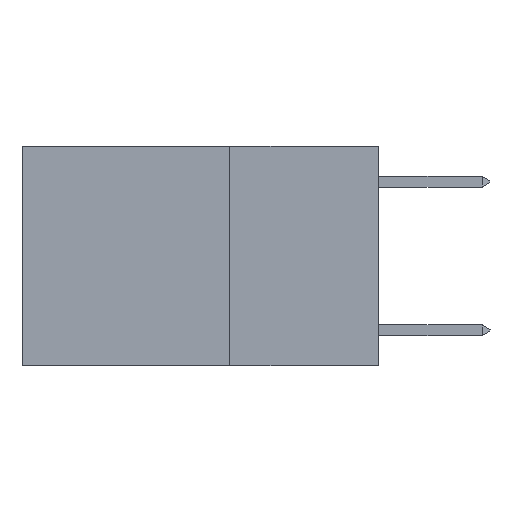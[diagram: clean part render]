
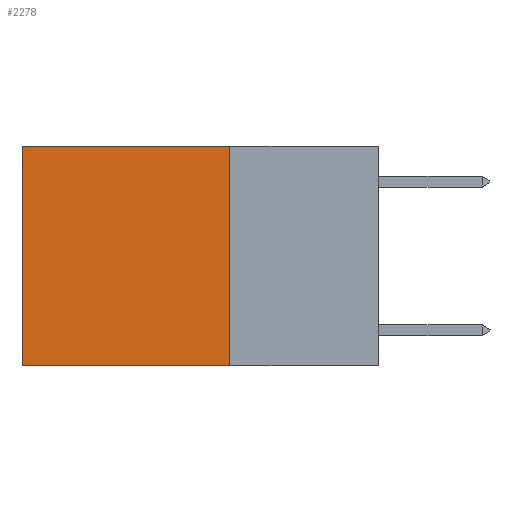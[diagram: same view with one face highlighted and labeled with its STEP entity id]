
A CAD part, left-side view. The second image highlights one B-rep face of the part: STEP entity #2278.
In plain terms, the highlighted planar face has unit normal (-1, 0, 0).
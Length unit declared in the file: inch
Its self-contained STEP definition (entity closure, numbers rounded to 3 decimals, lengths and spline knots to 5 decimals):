
#2278 = ADVANCED_FACE ( 'NONE', ( #11460 ), #9833, .F. ) ;
#2543 = EDGE_CURVE ( 'NONE', #5495, #20544, #8423, .T. ) ;
#2946 = DIRECTION ( 'NONE',  ( 1., 0., 0. ) ) ;
#3876 = DIRECTION ( 'NONE',  ( 0., 1., 0. ) ) ;
#5283 = DIRECTION ( 'NONE',  ( 0., 0., -1. ) ) ;
#5495 = VERTEX_POINT ( 'NONE', #20802 ) ;
#7381 = ORIENTED_EDGE ( 'NONE', *, *, #27551, .T. ) ;
#7865 = VERTEX_POINT ( 'NONE', #26827 ) ;
#8309 = VECTOR ( 'NONE', #28486, 39.37008 ) ;
#8423 = LINE ( 'NONE', #19993, #8309 ) ;
#9833 = PLANE ( 'NONE',  #25409 ) ;
#10923 = EDGE_CURVE ( 'NONE', #26801, #5495, #21023, .T. ) ;
#11460 = FACE_OUTER_BOUND ( 'NONE', #23598, .T. ) ;
#13222 = CARTESIAN_POINT ( 'NONE',  ( 0.2625, 0.6, -0.37 ) ) ;
#13610 = VECTOR ( 'NONE', #3876, 39.37008 ) ;
#13968 = LINE ( 'NONE', #26446, #13610 ) ;
#15145 = LINE ( 'NONE', #16872, #25514 ) ;
#16305 = EDGE_CURVE ( 'NONE', #26801, #7865, #13968, .T. ) ;
#16872 = CARTESIAN_POINT ( 'NONE',  ( 0.2625, 0.6, 0. ) ) ;
#19121 = DIRECTION ( 'NONE',  ( 0., 0., -1. ) ) ;
#19144 = CARTESIAN_POINT ( 'NONE',  ( 0.2625, 0.25, 0. ) ) ;
#19270 = ORIENTED_EDGE ( 'NONE', *, *, #16305, .T. ) ;
#19993 = CARTESIAN_POINT ( 'NONE',  ( 0.2625, 0.25, -0.37 ) ) ;
#20544 = VERTEX_POINT ( 'NONE', #13222 ) ;
#20721 = VECTOR ( 'NONE', #5283, 39.37008 ) ;
#20802 = CARTESIAN_POINT ( 'NONE',  ( 0.2625, 0.25, -0.37 ) ) ;
#21023 = LINE ( 'NONE', #19144, #20721 ) ;
#21544 = ORIENTED_EDGE ( 'NONE', *, *, #2543, .F. ) ;
#23515 = DIRECTION ( 'NONE',  ( 0., 0., -1. ) ) ;
#23598 = EDGE_LOOP ( 'NONE', ( #7381, #21544, #24295, #19270 ) ) ;
#24295 = ORIENTED_EDGE ( 'NONE', *, *, #10923, .F. ) ;
#25090 = CARTESIAN_POINT ( 'NONE',  ( 0.2625, 0.25, 0. ) ) ;
#25409 = AXIS2_PLACEMENT_3D ( 'NONE', #27685, #2946, #19121 ) ;
#25514 = VECTOR ( 'NONE', #23515, 39.37008 ) ;
#26446 = CARTESIAN_POINT ( 'NONE',  ( 0.2625, 0.25, 0. ) ) ;
#26801 = VERTEX_POINT ( 'NONE', #25090 ) ;
#26827 = CARTESIAN_POINT ( 'NONE',  ( 0.2625, 0.6, 0. ) ) ;
#27551 = EDGE_CURVE ( 'NONE', #7865, #20544, #15145, .T. ) ;
#27685 = CARTESIAN_POINT ( 'NONE',  ( 0.2625, 0.25, 0. ) ) ;
#28486 = DIRECTION ( 'NONE',  ( 0., 1., 0. ) ) ;
